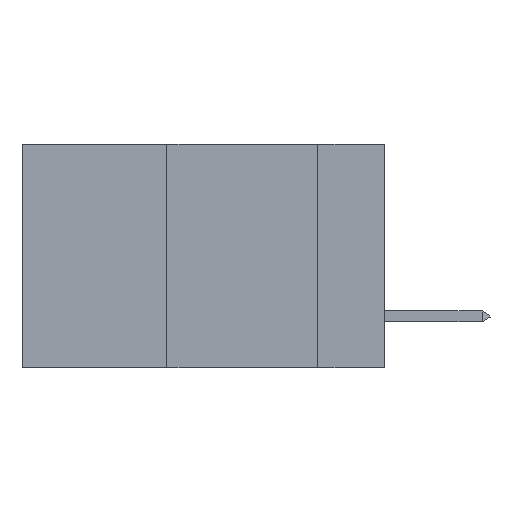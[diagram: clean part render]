
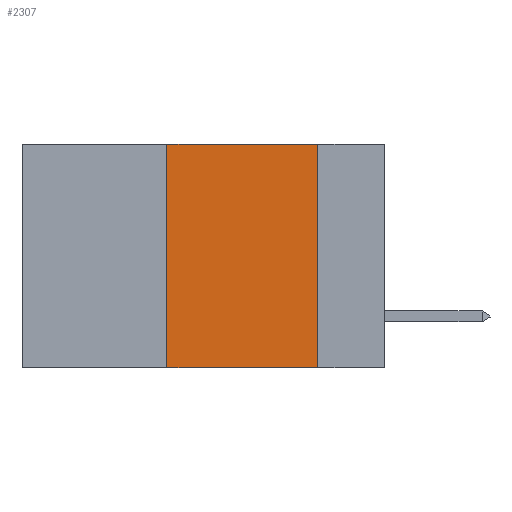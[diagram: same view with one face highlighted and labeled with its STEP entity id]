
A CAD part, left-side view. The second image highlights one B-rep face of the part: STEP entity #2307.
In plain terms, the highlighted planar face has unit normal (-1, 0, 0).
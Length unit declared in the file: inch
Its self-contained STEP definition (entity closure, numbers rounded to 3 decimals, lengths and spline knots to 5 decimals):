
#194 = CARTESIAN_POINT ( 'NONE',  ( 0., 0.36, 0. ) ) ;
#1104 = DIRECTION ( 'NONE',  ( 0., -1., 0. ) ) ;
#1850 = VECTOR ( 'NONE', #1104, 39.37008 ) ;
#2032 = AXIS2_PLACEMENT_3D ( 'NONE', #10008, #22360, #13300 ) ;
#2307 = ADVANCED_FACE ( 'NONE', ( #4259 ), #20463, .F. ) ;
#3962 = DIRECTION ( 'NONE',  ( 0., -1., 0. ) ) ;
#4259 = FACE_OUTER_BOUND ( 'NONE', #9792, .T. ) ;
#4522 = VERTEX_POINT ( 'NONE', #194 ) ;
#4570 = LINE ( 'NONE', #14778, #1850 ) ;
#6274 = ORIENTED_EDGE ( 'NONE', *, *, #11545, .F. ) ;
#7587 = LINE ( 'NONE', #18455, #17992 ) ;
#7958 = DIRECTION ( 'NONE',  ( 0., 0., -1. ) ) ;
#8120 = EDGE_CURVE ( 'NONE', #18379, #11129, #4570, .T. ) ;
#9792 = EDGE_LOOP ( 'NONE', ( #6274, #11568, #13651, #12586 ) ) ;
#10008 = CARTESIAN_POINT ( 'NONE',  ( 0., 0.6, 0. ) ) ;
#10864 = CARTESIAN_POINT ( 'NONE',  ( 0., 0.6, 0. ) ) ;
#11129 = VERTEX_POINT ( 'NONE', #21994 ) ;
#11194 = CARTESIAN_POINT ( 'NONE',  ( 0., 0.36, -0.37 ) ) ;
#11545 = EDGE_CURVE ( 'NONE', #14034, #11129, #7587, .T. ) ;
#11568 = ORIENTED_EDGE ( 'NONE', *, *, #12606, .F. ) ;
#12027 = CARTESIAN_POINT ( 'NONE',  ( 0., 0.11, 0. ) ) ;
#12586 = ORIENTED_EDGE ( 'NONE', *, *, #8120, .T. ) ;
#12606 = EDGE_CURVE ( 'NONE', #4522, #14034, #22042, .T. ) ;
#13300 = DIRECTION ( 'NONE',  ( 0., 0., -1. ) ) ;
#13651 = ORIENTED_EDGE ( 'NONE', *, *, #22556, .F. ) ;
#14034 = VERTEX_POINT ( 'NONE', #12027 ) ;
#14778 = CARTESIAN_POINT ( 'NONE',  ( 0., 0.6, -0.37 ) ) ;
#16116 = DIRECTION ( 'NONE',  ( 0., 0., 1. ) ) ;
#17406 = VECTOR ( 'NONE', #3962, 39.37008 ) ;
#17820 = CARTESIAN_POINT ( 'NONE',  ( 0., 0.36, 0. ) ) ;
#17992 = VECTOR ( 'NONE', #7958, 39.37008 ) ;
#18379 = VERTEX_POINT ( 'NONE', #11194 ) ;
#18455 = CARTESIAN_POINT ( 'NONE',  ( 0., 0.11, 0. ) ) ;
#20463 = PLANE ( 'NONE',  #2032 ) ;
#21898 = VECTOR ( 'NONE', #16116, 39.37008 ) ;
#21994 = CARTESIAN_POINT ( 'NONE',  ( 0., 0.11, -0.37 ) ) ;
#22042 = LINE ( 'NONE', #10864, #17406 ) ;
#22360 = DIRECTION ( 'NONE',  ( 1., 0., 0. ) ) ;
#22449 = LINE ( 'NONE', #17820, #21898 ) ;
#22556 = EDGE_CURVE ( 'NONE', #18379, #4522, #22449, .T. ) ;
